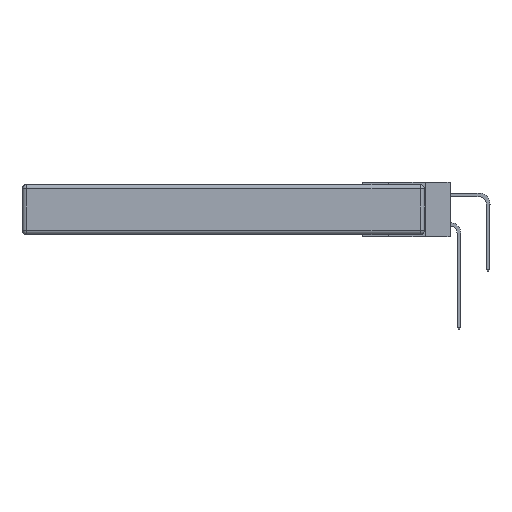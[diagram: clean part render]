
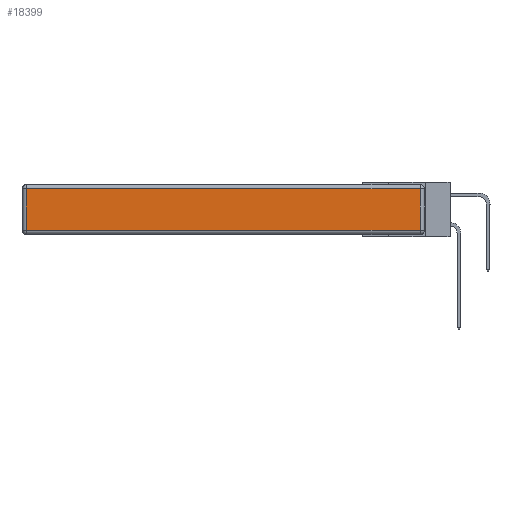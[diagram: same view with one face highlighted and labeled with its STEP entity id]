
A CAD part, left-side view. The second image highlights one B-rep face of the part: STEP entity #18399.
In plain terms, the highlighted planar face has unit normal (-1, 0, 0).
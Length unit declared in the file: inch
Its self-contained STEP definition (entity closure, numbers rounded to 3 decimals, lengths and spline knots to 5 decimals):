
#593 = VECTOR ( 'NONE', #17496, 39.37008 ) ;
#1395 = ORIENTED_EDGE ( 'NONE', *, *, #9605, .T. ) ;
#1491 = VECTOR ( 'NONE', #17088, 39.37008 ) ;
#3077 = CARTESIAN_POINT ( 'NONE',  ( 0., 2.72, -0.03 ) ) ;
#5658 = FACE_OUTER_BOUND ( 'NONE', #29628, .T. ) ;
#6660 = CARTESIAN_POINT ( 'NONE',  ( 0., 2.72, -0.313 ) ) ;
#7664 = VERTEX_POINT ( 'NONE', #3077 ) ;
#8472 = LINE ( 'NONE', #14188, #593 ) ;
#8766 = ORIENTED_EDGE ( 'NONE', *, *, #28128, .T. ) ;
#9127 = PLANE ( 'NONE',  #31566 ) ;
#9458 = EDGE_CURVE ( 'NONE', #7664, #27804, #18103, .T. ) ;
#9605 = EDGE_CURVE ( 'NONE', #27804, #20256, #15704, .T. ) ;
#14188 = CARTESIAN_POINT ( 'NONE',  ( 0., 2.75, -0.03 ) ) ;
#15704 = LINE ( 'NONE', #19406, #1491 ) ;
#16444 = CARTESIAN_POINT ( 'NONE',  ( 0., 2.72, -0.343 ) ) ;
#17088 = DIRECTION ( 'NONE',  ( 0., -1., 0. ) ) ;
#17496 = DIRECTION ( 'NONE',  ( 0., 1., 0. ) ) ;
#17818 = CARTESIAN_POINT ( 'NONE',  ( 0., 0.03, -0.343 ) ) ;
#18103 = LINE ( 'NONE', #16444, #31136 ) ;
#18399 = ADVANCED_FACE ( 'NONE', ( #5658 ), #9127, .T. ) ;
#19190 = CARTESIAN_POINT ( 'NONE',  ( 0., 0., -0.343 ) ) ;
#19406 = CARTESIAN_POINT ( 'NONE',  ( 0., 0., -0.313 ) ) ;
#19826 = CARTESIAN_POINT ( 'NONE',  ( 0., 0.03, -0.313 ) ) ;
#20256 = VERTEX_POINT ( 'NONE', #19826 ) ;
#20700 = DIRECTION ( 'NONE',  ( 0., 0., 1. ) ) ;
#23641 = LINE ( 'NONE', #17818, #30377 ) ;
#23989 = EDGE_CURVE ( 'NONE', #32241, #7664, #8472, .T. ) ;
#26180 = ORIENTED_EDGE ( 'NONE', *, *, #23989, .T. ) ;
#26716 = DIRECTION ( 'NONE',  ( 0., 0., 1. ) ) ;
#27804 = VERTEX_POINT ( 'NONE', #6660 ) ;
#28128 = EDGE_CURVE ( 'NONE', #20256, #32241, #23641, .T. ) ;
#29247 = DIRECTION ( 'NONE',  ( -1., 0., 0. ) ) ;
#29259 = DIRECTION ( 'NONE',  ( 0., 0., -1. ) ) ;
#29628 = EDGE_LOOP ( 'NONE', ( #1395, #8766, #26180, #29880 ) ) ;
#29657 = CARTESIAN_POINT ( 'NONE',  ( 0., 0.03, -0.03 ) ) ;
#29880 = ORIENTED_EDGE ( 'NONE', *, *, #9458, .T. ) ;
#30377 = VECTOR ( 'NONE', #20700, 39.37008 ) ;
#31136 = VECTOR ( 'NONE', #29259, 39.37008 ) ;
#31566 = AXIS2_PLACEMENT_3D ( 'NONE', #19190, #29247, #26716 ) ;
#32241 = VERTEX_POINT ( 'NONE', #29657 ) ;
